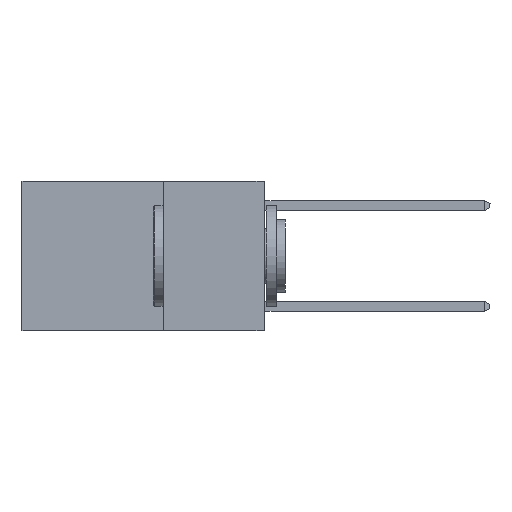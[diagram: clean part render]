
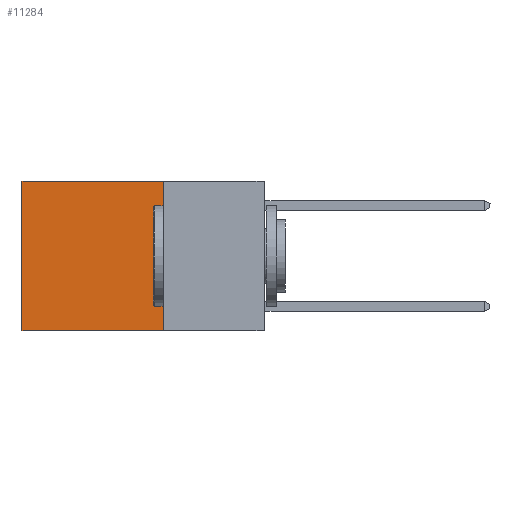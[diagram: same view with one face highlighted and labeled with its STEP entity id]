
A CAD part, left-side view. The second image highlights one B-rep face of the part: STEP entity #11284.
In plain terms, the highlighted planar face has unit normal (-1, 0, 0).
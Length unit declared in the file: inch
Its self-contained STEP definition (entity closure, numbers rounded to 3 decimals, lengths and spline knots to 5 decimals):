
#768 = DIRECTION ( 'NONE',  ( 0., 0., -1. ) ) ;
#894 = CARTESIAN_POINT ( 'NONE',  ( 0.2625, 0.25, 0. ) ) ;
#923 = VERTEX_POINT ( 'NONE', #12041 ) ;
#2243 = CARTESIAN_POINT ( 'NONE',  ( 0.2625, 0.25, -0.37 ) ) ;
#2478 = DIRECTION ( 'NONE',  ( 0., 0., -1. ) ) ;
#3013 = LINE ( 'NONE', #2243, #15073 ) ;
#3146 = CARTESIAN_POINT ( 'NONE',  ( 0.2625, 0.6, 0. ) ) ;
#3161 = FACE_OUTER_BOUND ( 'NONE', #4485, .T. ) ;
#3654 = EDGE_CURVE ( 'NONE', #8937, #7401, #14315, .T. ) ;
#4216 = EDGE_CURVE ( 'NONE', #923, #7401, #3013, .T. ) ;
#4485 = EDGE_LOOP ( 'NONE', ( #10386, #10172, #7321, #12622 ) ) ;
#4914 = VECTOR ( 'NONE', #11268, 39.37008 ) ;
#6243 = VECTOR ( 'NONE', #768, 39.37008 ) ;
#7143 = LINE ( 'NONE', #894, #4914 ) ;
#7152 = CARTESIAN_POINT ( 'NONE',  ( 0.2625, 0.25, 0. ) ) ;
#7321 = ORIENTED_EDGE ( 'NONE', *, *, #13593, .F. ) ;
#7401 = VERTEX_POINT ( 'NONE', #15898 ) ;
#8166 = CARTESIAN_POINT ( 'NONE',  ( 0.2625, 0.25, 0. ) ) ;
#8255 = DIRECTION ( 'NONE',  ( 1., 0., 0. ) ) ;
#8290 = VECTOR ( 'NONE', #8399, 39.37008 ) ;
#8399 = DIRECTION ( 'NONE',  ( 0., 1., 0. ) ) ;
#8937 = VERTEX_POINT ( 'NONE', #11629 ) ;
#9606 = CARTESIAN_POINT ( 'NONE',  ( 0.2625, 0.25, 0. ) ) ;
#9777 = DIRECTION ( 'NONE',  ( 0., 1., 0. ) ) ;
#10172 = ORIENTED_EDGE ( 'NONE', *, *, #4216, .F. ) ;
#10386 = ORIENTED_EDGE ( 'NONE', *, *, #3654, .T. ) ;
#10829 = LINE ( 'NONE', #9606, #8290 ) ;
#11098 = AXIS2_PLACEMENT_3D ( 'NONE', #8166, #8255, #2478 ) ;
#11268 = DIRECTION ( 'NONE',  ( 0., 0., -1. ) ) ;
#11284 = ADVANCED_FACE ( 'NONE', ( #3161 ), #14404, .F. ) ;
#11629 = CARTESIAN_POINT ( 'NONE',  ( 0.2625, 0.6, 0. ) ) ;
#12041 = CARTESIAN_POINT ( 'NONE',  ( 0.2625, 0.25, -0.37 ) ) ;
#12622 = ORIENTED_EDGE ( 'NONE', *, *, #13119, .T. ) ;
#13119 = EDGE_CURVE ( 'NONE', #15618, #8937, #10829, .T. ) ;
#13593 = EDGE_CURVE ( 'NONE', #15618, #923, #7143, .T. ) ;
#14315 = LINE ( 'NONE', #3146, #6243 ) ;
#14404 = PLANE ( 'NONE',  #11098 ) ;
#15073 = VECTOR ( 'NONE', #9777, 39.37008 ) ;
#15618 = VERTEX_POINT ( 'NONE', #7152 ) ;
#15898 = CARTESIAN_POINT ( 'NONE',  ( 0.2625, 0.6, -0.37 ) ) ;
